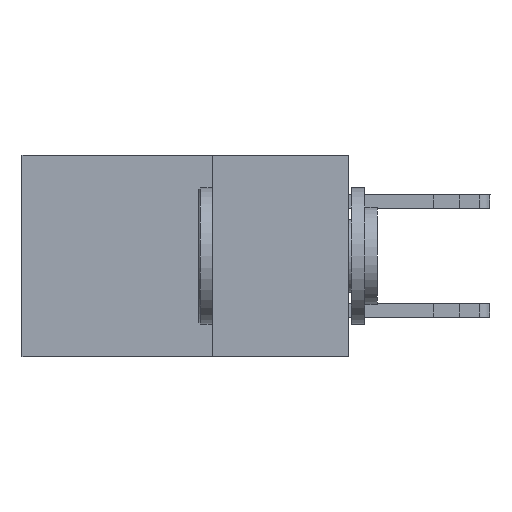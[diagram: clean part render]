
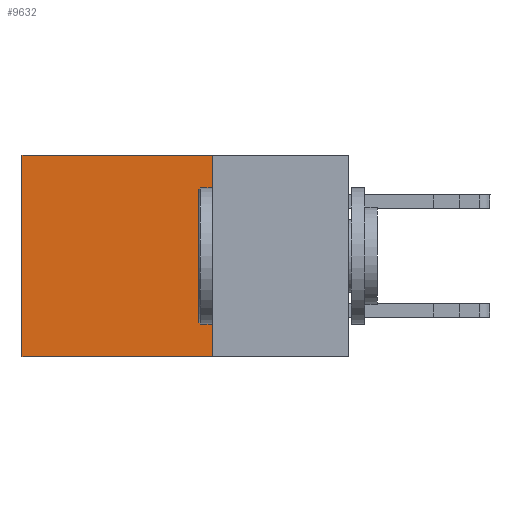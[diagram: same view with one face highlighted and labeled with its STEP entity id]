
A CAD part, left-side view. The second image highlights one B-rep face of the part: STEP entity #9632.
In plain terms, the highlighted planar face has unit normal (-1, 0, 0).
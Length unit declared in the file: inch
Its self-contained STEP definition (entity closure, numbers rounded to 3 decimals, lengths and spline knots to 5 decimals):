
#348 = VERTEX_POINT ( 'NONE', #742 ) ;
#403 = EDGE_CURVE ( 'NONE', #8819, #348, #7497, .T. ) ;
#742 = CARTESIAN_POINT ( 'NONE',  ( 0.298, 0.6, 0. ) ) ;
#1347 = VERTEX_POINT ( 'NONE', #12836 ) ;
#1365 = VECTOR ( 'NONE', #9100, 39.37008 ) ;
#1690 = VECTOR ( 'NONE', #2306, 39.37008 ) ;
#2007 = DIRECTION ( 'NONE',  ( 0., 0., -1. ) ) ;
#2221 = DIRECTION ( 'NONE',  ( 1., 0., 0. ) ) ;
#2306 = DIRECTION ( 'NONE',  ( 0., 0., -1. ) ) ;
#2676 = CARTESIAN_POINT ( 'NONE',  ( 0.298, 0.25, 0. ) ) ;
#3689 = ORIENTED_EDGE ( 'NONE', *, *, #403, .T. ) ;
#5065 = EDGE_CURVE ( 'NONE', #8819, #10258, #8368, .T. ) ;
#5552 = EDGE_CURVE ( 'NONE', #10258, #1347, #10560, .T. ) ;
#6280 = VECTOR ( 'NONE', #13739, 39.37008 ) ;
#7497 = LINE ( 'NONE', #2676, #1365 ) ;
#8368 = LINE ( 'NONE', #18448, #14028 ) ;
#8819 = VERTEX_POINT ( 'NONE', #12199 ) ;
#9100 = DIRECTION ( 'NONE',  ( 0., 1., 0. ) ) ;
#9632 = ADVANCED_FACE ( 'NONE', ( #13420 ), #11615, .F. ) ;
#10258 = VERTEX_POINT ( 'NONE', #19388 ) ;
#10560 = LINE ( 'NONE', #13841, #6280 ) ;
#11615 = PLANE ( 'NONE',  #18707 ) ;
#12199 = CARTESIAN_POINT ( 'NONE',  ( 0.298, 0.25, 0. ) ) ;
#12836 = CARTESIAN_POINT ( 'NONE',  ( 0.298, 0.6, -0.37 ) ) ;
#12884 = ORIENTED_EDGE ( 'NONE', *, *, #14219, .T. ) ;
#13067 = ORIENTED_EDGE ( 'NONE', *, *, #5065, .F. ) ;
#13420 = FACE_OUTER_BOUND ( 'NONE', #14942, .T. ) ;
#13739 = DIRECTION ( 'NONE',  ( 0., 1., 0. ) ) ;
#13841 = CARTESIAN_POINT ( 'NONE',  ( 0.298, 0.25, -0.37 ) ) ;
#14028 = VECTOR ( 'NONE', #19605, 39.37008 ) ;
#14219 = EDGE_CURVE ( 'NONE', #348, #1347, #14873, .T. ) ;
#14873 = LINE ( 'NONE', #20185, #1690 ) ;
#14942 = EDGE_LOOP ( 'NONE', ( #12884, #18750, #13067, #3689 ) ) ;
#18069 = CARTESIAN_POINT ( 'NONE',  ( 0.298, 0.25, 0. ) ) ;
#18448 = CARTESIAN_POINT ( 'NONE',  ( 0.298, 0.25, 0. ) ) ;
#18707 = AXIS2_PLACEMENT_3D ( 'NONE', #18069, #2221, #2007 ) ;
#18750 = ORIENTED_EDGE ( 'NONE', *, *, #5552, .F. ) ;
#19388 = CARTESIAN_POINT ( 'NONE',  ( 0.298, 0.25, -0.37 ) ) ;
#19605 = DIRECTION ( 'NONE',  ( 0., 0., -1. ) ) ;
#20185 = CARTESIAN_POINT ( 'NONE',  ( 0.298, 0.6, 0. ) ) ;
